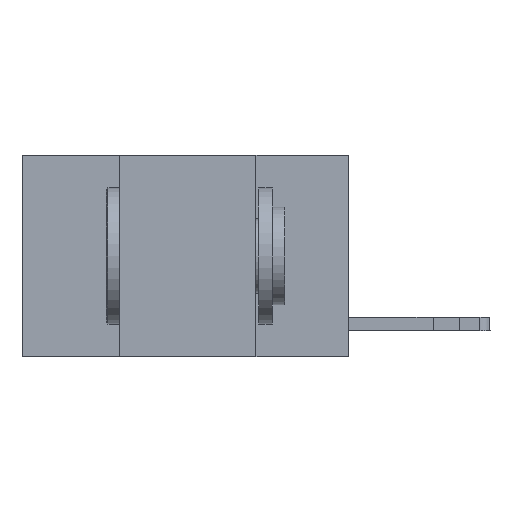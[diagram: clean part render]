
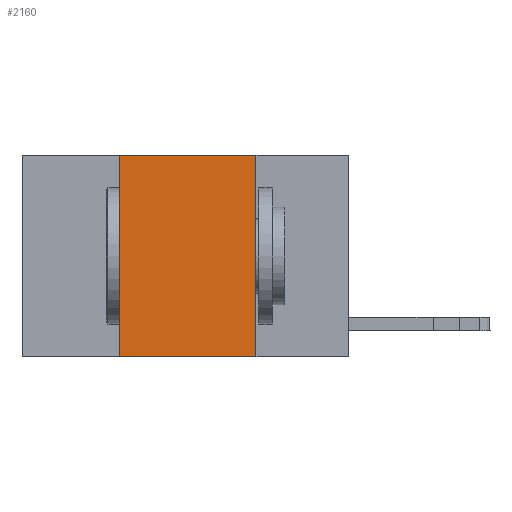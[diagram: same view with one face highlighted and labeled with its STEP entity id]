
A CAD part, left-side view. The second image highlights one B-rep face of the part: STEP entity #2160.
In plain terms, the highlighted planar face has unit normal (-1, 0, 0).
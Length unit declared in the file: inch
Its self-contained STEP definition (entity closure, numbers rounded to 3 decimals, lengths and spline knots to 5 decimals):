
#24 = VECTOR ( 'NONE', #9973, 39.37008 ) ;
#534 = AXIS2_PLACEMENT_3D ( 'NONE', #7202, #7184, #7120 ) ;
#823 = EDGE_LOOP ( 'NONE', ( #843, #9091, #11875, #1809 ) ) ;
#843 = ORIENTED_EDGE ( 'NONE', *, *, #9896, .F. ) ;
#1307 = CARTESIAN_POINT ( 'NONE',  ( 0., 0.6, -0.37 ) ) ;
#1809 = ORIENTED_EDGE ( 'NONE', *, *, #4057, .T. ) ;
#1836 = CARTESIAN_POINT ( 'NONE',  ( 0., 0.17, 0. ) ) ;
#1922 = LINE ( 'NONE', #10020, #6939 ) ;
#2160 = ADVANCED_FACE ( 'NONE', ( #8972 ), #7458, .F. ) ;
#2742 = VECTOR ( 'NONE', #11144, 39.37008 ) ;
#3222 = VECTOR ( 'NONE', #5042, 39.37008 ) ;
#3559 = VERTEX_POINT ( 'NONE', #9255 ) ;
#3957 = EDGE_CURVE ( 'NONE', #12032, #8180, #1922, .T. ) ;
#4057 = EDGE_CURVE ( 'NONE', #8967, #3559, #8004, .T. ) ;
#4649 = LINE ( 'NONE', #7944, #3222 ) ;
#5042 = DIRECTION ( 'NONE',  ( 0., 0., -1. ) ) ;
#6939 = VECTOR ( 'NONE', #10981, 39.37008 ) ;
#7120 = DIRECTION ( 'NONE',  ( 0., 0., -1. ) ) ;
#7184 = DIRECTION ( 'NONE',  ( 1., 0., 0. ) ) ;
#7202 = CARTESIAN_POINT ( 'NONE',  ( 0., 0.6, 0. ) ) ;
#7458 = PLANE ( 'NONE',  #534 ) ;
#7944 = CARTESIAN_POINT ( 'NONE',  ( 0., 0.17, 0. ) ) ;
#8004 = LINE ( 'NONE', #1307, #2742 ) ;
#8180 = VERTEX_POINT ( 'NONE', #1836 ) ;
#8967 = VERTEX_POINT ( 'NONE', #11812 ) ;
#8972 = FACE_OUTER_BOUND ( 'NONE', #823, .T. ) ;
#9091 = ORIENTED_EDGE ( 'NONE', *, *, #3957, .F. ) ;
#9255 = CARTESIAN_POINT ( 'NONE',  ( 0., 0.17, -0.37 ) ) ;
#9842 = CARTESIAN_POINT ( 'NONE',  ( 0., 0.42, 0. ) ) ;
#9896 = EDGE_CURVE ( 'NONE', #8180, #3559, #4649, .T. ) ;
#9973 = DIRECTION ( 'NONE',  ( 0., 0., 1. ) ) ;
#10020 = CARTESIAN_POINT ( 'NONE',  ( 0., 0.6, 0. ) ) ;
#10285 = LINE ( 'NONE', #11854, #24 ) ;
#10981 = DIRECTION ( 'NONE',  ( 0., -1., 0. ) ) ;
#11144 = DIRECTION ( 'NONE',  ( 0., -1., 0. ) ) ;
#11812 = CARTESIAN_POINT ( 'NONE',  ( 0., 0.42, -0.37 ) ) ;
#11854 = CARTESIAN_POINT ( 'NONE',  ( 0., 0.42, 0. ) ) ;
#11875 = ORIENTED_EDGE ( 'NONE', *, *, #12147, .F. ) ;
#12032 = VERTEX_POINT ( 'NONE', #9842 ) ;
#12147 = EDGE_CURVE ( 'NONE', #8967, #12032, #10285, .T. ) ;
